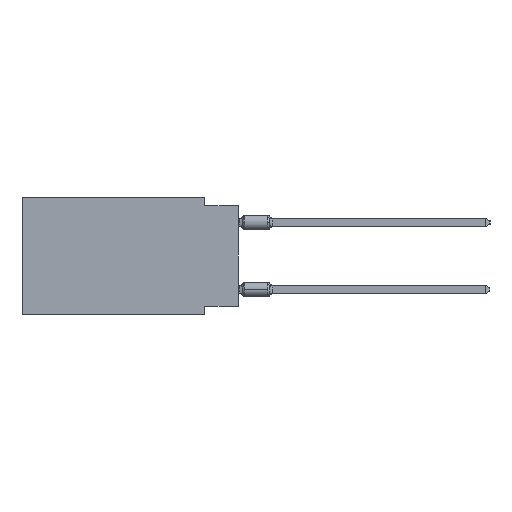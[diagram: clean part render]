
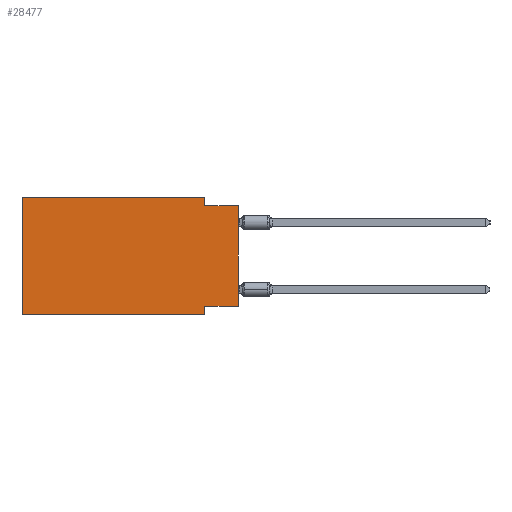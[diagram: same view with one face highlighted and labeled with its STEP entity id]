
A CAD part, left-side view. The second image highlights one B-rep face of the part: STEP entity #28477.
In plain terms, the highlighted planar face has unit normal (-1, 0, 0).
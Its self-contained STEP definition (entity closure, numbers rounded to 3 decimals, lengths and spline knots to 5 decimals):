
#1941 = VECTOR ( 'NONE', #4012, 39.37008 ) ;
#4012 = DIRECTION ( 'NONE',  ( 0., 1., 0. ) ) ;
#4082 = CARTESIAN_POINT ( 'NONE',  ( 0., 0.1, 0. ) ) ;
#4826 = EDGE_CURVE ( 'NONE', #54949, #21698, #10560, .T. ) ;
#5900 = EDGE_CURVE ( 'NONE', #27610, #50929, #31601, .T. ) ;
#5993 = CARTESIAN_POINT ( 'NONE',  ( 0., 0.645, 0. ) ) ;
#6818 = DIRECTION ( 'NONE',  ( 0., -1., 0. ) ) ;
#7729 = VERTEX_POINT ( 'NONE', #32175 ) ;
#9651 = ORIENTED_EDGE ( 'NONE', *, *, #44368, .F. ) ;
#9736 = DIRECTION ( 'NONE',  ( 0., 0., 1. ) ) ;
#10560 = LINE ( 'NONE', #15996, #36042 ) ;
#10787 = VECTOR ( 'NONE', #23646, 39.37008 ) ;
#11254 = LINE ( 'NONE', #15010, #10787 ) ;
#11284 = EDGE_CURVE ( 'NONE', #44065, #21698, #55251, .T. ) ;
#12431 = CARTESIAN_POINT ( 'NONE',  ( 0., 0.645, 0. ) ) ;
#14125 = CARTESIAN_POINT ( 'NONE',  ( 0., 0., -0.325 ) ) ;
#14489 = EDGE_CURVE ( 'NONE', #27610, #17649, #38284, .T. ) ;
#15010 = CARTESIAN_POINT ( 'NONE',  ( 0., 0.1, -0.35 ) ) ;
#15608 = DIRECTION ( 'NONE',  ( 0., 0., 1. ) ) ;
#15996 = CARTESIAN_POINT ( 'NONE',  ( 0., 0., -0.025 ) ) ;
#17649 = VERTEX_POINT ( 'NONE', #36964 ) ;
#17666 = ORIENTED_EDGE ( 'NONE', *, *, #27685, .F. ) ;
#18094 = LINE ( 'NONE', #5993, #25078 ) ;
#18501 = ORIENTED_EDGE ( 'NONE', *, *, #4826, .F. ) ;
#19392 = FACE_OUTER_BOUND ( 'NONE', #54054, .T. ) ;
#21698 = VERTEX_POINT ( 'NONE', #33959 ) ;
#22174 = ORIENTED_EDGE ( 'NONE', *, *, #48952, .F. ) ;
#23208 = CARTESIAN_POINT ( 'NONE',  ( 0., 0.1, 0. ) ) ;
#23542 = DIRECTION ( 'NONE',  ( 0., -1., 0. ) ) ;
#23572 = CARTESIAN_POINT ( 'NONE',  ( 0., 0.1, -0.025 ) ) ;
#23646 = DIRECTION ( 'NONE',  ( 0., 0., -1. ) ) ;
#25078 = VECTOR ( 'NONE', #23542, 39.37008 ) ;
#27610 = VERTEX_POINT ( 'NONE', #45463 ) ;
#27685 = EDGE_CURVE ( 'NONE', #7729, #17649, #11254, .T. ) ;
#28477 = ADVANCED_FACE ( 'NONE', ( #19392 ), #36936, .F. ) ;
#28993 = ORIENTED_EDGE ( 'NONE', *, *, #11284, .T. ) ;
#29160 = CARTESIAN_POINT ( 'NONE',  ( 0., 0.645, 0. ) ) ;
#29227 = ORIENTED_EDGE ( 'NONE', *, *, #48528, .F. ) ;
#29415 = DIRECTION ( 'NONE',  ( 0., -1., 0. ) ) ;
#30141 = AXIS2_PLACEMENT_3D ( 'NONE', #29160, #37769, #54447 ) ;
#31601 = LINE ( 'NONE', #36195, #48176 ) ;
#32175 = CARTESIAN_POINT ( 'NONE',  ( 0., 0.1, -0.325 ) ) ;
#33959 = CARTESIAN_POINT ( 'NONE',  ( 0., 0., -0.025 ) ) ;
#35169 = VERTEX_POINT ( 'NONE', #4082 ) ;
#35290 = LINE ( 'NONE', #23208, #40617 ) ;
#36042 = VECTOR ( 'NONE', #6818, 39.37008 ) ;
#36195 = CARTESIAN_POINT ( 'NONE',  ( 0., 0.645, 0. ) ) ;
#36936 = PLANE ( 'NONE',  #30141 ) ;
#36964 = CARTESIAN_POINT ( 'NONE',  ( 0., 0.1, -0.35 ) ) ;
#37769 = DIRECTION ( 'NONE',  ( 1., 0., 0. ) ) ;
#38284 = LINE ( 'NONE', #54694, #53399 ) ;
#39644 = LINE ( 'NONE', #43380, #1941 ) ;
#40617 = VECTOR ( 'NONE', #43885, 39.37008 ) ;
#43380 = CARTESIAN_POINT ( 'NONE',  ( 0., 0., -0.325 ) ) ;
#43885 = DIRECTION ( 'NONE',  ( 0., 0., -1. ) ) ;
#44065 = VERTEX_POINT ( 'NONE', #14125 ) ;
#44368 = EDGE_CURVE ( 'NONE', #44065, #7729, #39644, .T. ) ;
#45463 = CARTESIAN_POINT ( 'NONE',  ( 0., 0.645, -0.35 ) ) ;
#46332 = CARTESIAN_POINT ( 'NONE',  ( 0., 0., 0. ) ) ;
#46999 = ORIENTED_EDGE ( 'NONE', *, *, #5900, .F. ) ;
#48176 = VECTOR ( 'NONE', #9736, 39.37008 ) ;
#48528 = EDGE_CURVE ( 'NONE', #50929, #35169, #18094, .T. ) ;
#48952 = EDGE_CURVE ( 'NONE', #35169, #54949, #35290, .T. ) ;
#50929 = VERTEX_POINT ( 'NONE', #12431 ) ;
#52372 = VECTOR ( 'NONE', #15608, 39.37008 ) ;
#53399 = VECTOR ( 'NONE', #29415, 39.37008 ) ;
#54054 = EDGE_LOOP ( 'NONE', ( #28993, #18501, #22174, #29227, #46999, #55920, #17666, #9651 ) ) ;
#54447 = DIRECTION ( 'NONE',  ( 0., 0., -1. ) ) ;
#54694 = CARTESIAN_POINT ( 'NONE',  ( 0., 0.645, -0.35 ) ) ;
#54949 = VERTEX_POINT ( 'NONE', #23572 ) ;
#55251 = LINE ( 'NONE', #46332, #52372 ) ;
#55920 = ORIENTED_EDGE ( 'NONE', *, *, #14489, .T. ) ;
